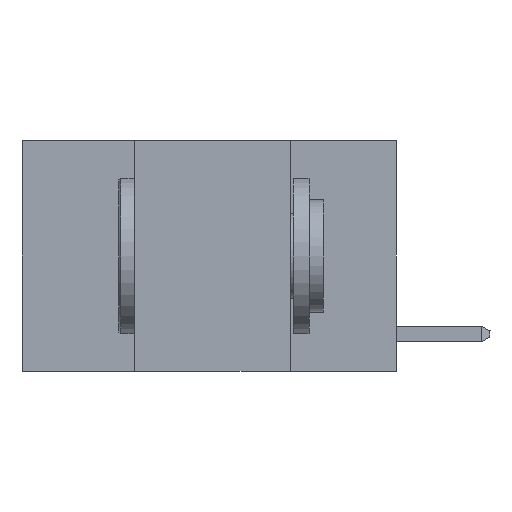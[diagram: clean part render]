
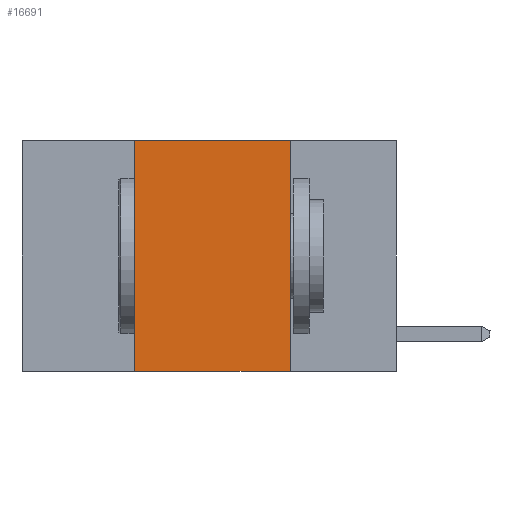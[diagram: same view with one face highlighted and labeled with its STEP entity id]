
A CAD part, left-side view. The second image highlights one B-rep face of the part: STEP entity #16691.
In plain terms, the highlighted planar face has unit normal (-1, 0, 0).
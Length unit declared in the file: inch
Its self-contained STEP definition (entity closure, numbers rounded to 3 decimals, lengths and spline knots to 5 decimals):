
#1723 = DIRECTION ( 'NONE',  ( 0., -1., 0. ) ) ;
#2367 = LINE ( 'NONE', #6729, #7058 ) ;
#3170 = VECTOR ( 'NONE', #26014, 39.37008 ) ;
#5045 = DIRECTION ( 'NONE',  ( 0., 0., 1. ) ) ;
#5328 = CARTESIAN_POINT ( 'NONE',  ( 0., 0.42, 0. ) ) ;
#5458 = EDGE_CURVE ( 'NONE', #24145, #9101, #14990, .T. ) ;
#6729 = CARTESIAN_POINT ( 'NONE',  ( 0., 0.17, 0. ) ) ;
#7058 = VECTOR ( 'NONE', #20555, 39.37008 ) ;
#7223 = EDGE_CURVE ( 'NONE', #27285, #16441, #20364, .T. ) ;
#7260 = LINE ( 'NONE', #16432, #16838 ) ;
#8040 = EDGE_CURVE ( 'NONE', #16441, #9101, #2367, .T. ) ;
#8406 = AXIS2_PLACEMENT_3D ( 'NONE', #26964, #15367, #10851 ) ;
#8599 = FACE_OUTER_BOUND ( 'NONE', #20387, .T. ) ;
#8979 = VECTOR ( 'NONE', #1723, 39.37008 ) ;
#9101 = VERTEX_POINT ( 'NONE', #21099 ) ;
#9211 = EDGE_CURVE ( 'NONE', #24145, #27285, #7260, .T. ) ;
#9338 = ORIENTED_EDGE ( 'NONE', *, *, #7223, .F. ) ;
#10737 = CARTESIAN_POINT ( 'NONE',  ( 0., 0.6, 0. ) ) ;
#10851 = DIRECTION ( 'NONE',  ( 0., 0., -1. ) ) ;
#12038 = ORIENTED_EDGE ( 'NONE', *, *, #8040, .F. ) ;
#12900 = ORIENTED_EDGE ( 'NONE', *, *, #5458, .T. ) ;
#14990 = LINE ( 'NONE', #28267, #3170 ) ;
#15367 = DIRECTION ( 'NONE',  ( 1., 0., 0. ) ) ;
#16432 = CARTESIAN_POINT ( 'NONE',  ( 0., 0.42, 0. ) ) ;
#16441 = VERTEX_POINT ( 'NONE', #23224 ) ;
#16691 = ADVANCED_FACE ( 'NONE', ( #8599 ), #17761, .F. ) ;
#16838 = VECTOR ( 'NONE', #5045, 39.37008 ) ;
#17761 = PLANE ( 'NONE',  #8406 ) ;
#20364 = LINE ( 'NONE', #10737, #8979 ) ;
#20387 = EDGE_LOOP ( 'NONE', ( #12038, #9338, #29036, #12900 ) ) ;
#20555 = DIRECTION ( 'NONE',  ( 0., 0., -1. ) ) ;
#21099 = CARTESIAN_POINT ( 'NONE',  ( 0., 0.17, -0.37 ) ) ;
#21173 = CARTESIAN_POINT ( 'NONE',  ( 0., 0.42, -0.37 ) ) ;
#23224 = CARTESIAN_POINT ( 'NONE',  ( 0., 0.17, 0. ) ) ;
#24145 = VERTEX_POINT ( 'NONE', #21173 ) ;
#26014 = DIRECTION ( 'NONE',  ( 0., -1., 0. ) ) ;
#26964 = CARTESIAN_POINT ( 'NONE',  ( 0., 0.6, 0. ) ) ;
#27285 = VERTEX_POINT ( 'NONE', #5328 ) ;
#28267 = CARTESIAN_POINT ( 'NONE',  ( 0., 0.6, -0.37 ) ) ;
#29036 = ORIENTED_EDGE ( 'NONE', *, *, #9211, .F. ) ;
